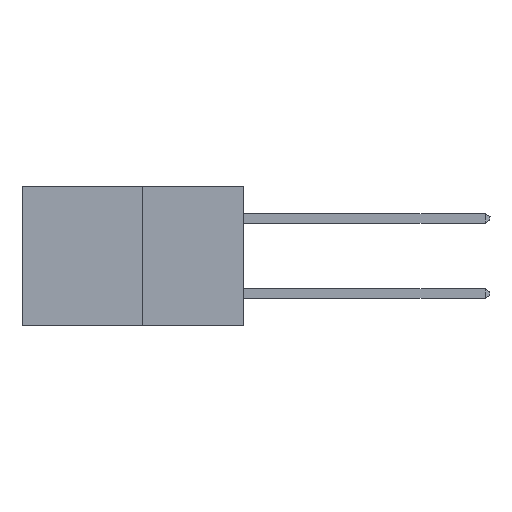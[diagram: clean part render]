
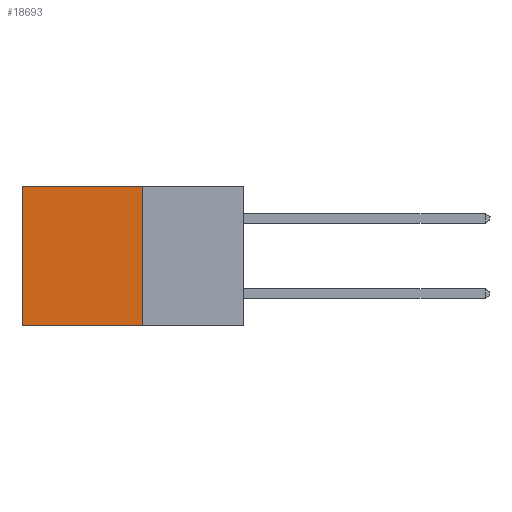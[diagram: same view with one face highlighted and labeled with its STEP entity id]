
A CAD part, left-side view. The second image highlights one B-rep face of the part: STEP entity #18693.
In plain terms, the highlighted planar face has unit normal (-1, 0, 0).
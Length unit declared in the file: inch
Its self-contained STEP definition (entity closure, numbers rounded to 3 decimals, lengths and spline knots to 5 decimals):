
#18 = ORIENTED_EDGE ( 'NONE', *, *, #7009, .T. ) ;
#288 = VECTOR ( 'NONE', #16341, 39.37008 ) ;
#577 = EDGE_CURVE ( 'NONE', #5076, #7932, #18253, .T. ) ;
#2026 = AXIS2_PLACEMENT_3D ( 'NONE', #16139, #15946, #15923 ) ;
#2952 = VECTOR ( 'NONE', #8415, 39.37008 ) ;
#3127 = CARTESIAN_POINT ( 'NONE',  ( 0.277, 0.27, 0. ) ) ;
#3936 = VECTOR ( 'NONE', #7826, 39.37008 ) ;
#4511 = CARTESIAN_POINT ( 'NONE',  ( 0.277, 0.59, -0.37 ) ) ;
#5076 = VERTEX_POINT ( 'NONE', #14349 ) ;
#5613 = EDGE_CURVE ( 'NONE', #15136, #7932, #16556, .T. ) ;
#6148 = VECTOR ( 'NONE', #7938, 39.37008 ) ;
#6212 = ORIENTED_EDGE ( 'NONE', *, *, #5613, .F. ) ;
#6992 = CARTESIAN_POINT ( 'NONE',  ( 0.277, 0.27, -0.37 ) ) ;
#7009 = EDGE_CURVE ( 'NONE', #16173, #5076, #8089, .T. ) ;
#7750 = CARTESIAN_POINT ( 'NONE',  ( 0.277, 0.27, 0. ) ) ;
#7826 = DIRECTION ( 'NONE',  ( 0., 1., 0. ) ) ;
#7932 = VERTEX_POINT ( 'NONE', #4511 ) ;
#7938 = DIRECTION ( 'NONE',  ( 0., 0., -1. ) ) ;
#8020 = EDGE_CURVE ( 'NONE', #16173, #15136, #14615, .T. ) ;
#8089 = LINE ( 'NONE', #3127, #3936 ) ;
#8415 = DIRECTION ( 'NONE',  ( 0., 0., -1. ) ) ;
#8995 = ORIENTED_EDGE ( 'NONE', *, *, #577, .T. ) ;
#10064 = CARTESIAN_POINT ( 'NONE',  ( 0.277, 0.27, -0.37 ) ) ;
#11607 = ORIENTED_EDGE ( 'NONE', *, *, #8020, .F. ) ;
#13007 = EDGE_LOOP ( 'NONE', ( #8995, #6212, #11607, #18 ) ) ;
#13550 = CARTESIAN_POINT ( 'NONE',  ( 0.277, 0.59, -0.37 ) ) ;
#14349 = CARTESIAN_POINT ( 'NONE',  ( 0.277, 0.59, 0. ) ) ;
#14615 = LINE ( 'NONE', #10064, #2952 ) ;
#14806 = FACE_OUTER_BOUND ( 'NONE', #13007, .T. ) ;
#15136 = VERTEX_POINT ( 'NONE', #17147 ) ;
#15923 = DIRECTION ( 'NONE',  ( 0., 0., -1. ) ) ;
#15946 = DIRECTION ( 'NONE',  ( 1., 0., 0. ) ) ;
#16139 = CARTESIAN_POINT ( 'NONE',  ( 0.277, 0.27, -0.37 ) ) ;
#16173 = VERTEX_POINT ( 'NONE', #7750 ) ;
#16189 = PLANE ( 'NONE',  #2026 ) ;
#16341 = DIRECTION ( 'NONE',  ( 0., 1., 0. ) ) ;
#16556 = LINE ( 'NONE', #6992, #288 ) ;
#17147 = CARTESIAN_POINT ( 'NONE',  ( 0.277, 0.27, -0.37 ) ) ;
#18253 = LINE ( 'NONE', #13550, #6148 ) ;
#18693 = ADVANCED_FACE ( 'NONE', ( #14806 ), #16189, .F. ) ;
